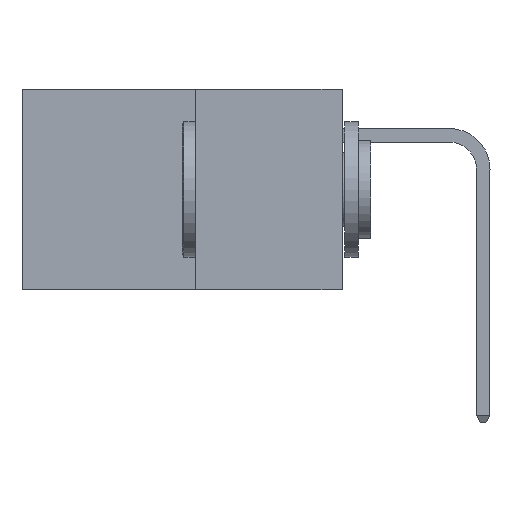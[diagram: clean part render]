
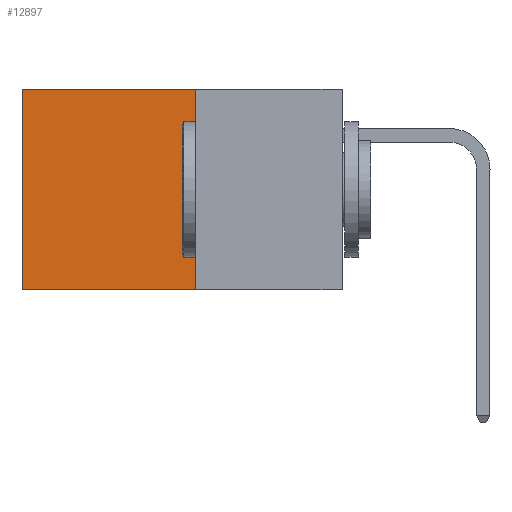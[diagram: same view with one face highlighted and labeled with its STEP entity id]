
A CAD part, left-side view. The second image highlights one B-rep face of the part: STEP entity #12897.
In plain terms, the highlighted planar face has unit normal (-1, 0, 0).
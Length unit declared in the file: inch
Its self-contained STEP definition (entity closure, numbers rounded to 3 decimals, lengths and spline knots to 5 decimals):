
#49 = EDGE_CURVE ( 'NONE', #3563, #13172, #6910, .T. ) ;
#600 = CARTESIAN_POINT ( 'NONE',  ( 0.277, 0.59, -0.37 ) ) ;
#800 = CARTESIAN_POINT ( 'NONE',  ( 0.277, 0.27, 0. ) ) ;
#1199 = ORIENTED_EDGE ( 'NONE', *, *, #7363, .F. ) ;
#1762 = LINE ( 'NONE', #2324, #5193 ) ;
#1766 = LINE ( 'NONE', #14304, #11670 ) ;
#1885 = AXIS2_PLACEMENT_3D ( 'NONE', #2661, #12996, #5249 ) ;
#2324 = CARTESIAN_POINT ( 'NONE',  ( 0.277, 0.27, -0.37 ) ) ;
#2379 = DIRECTION ( 'NONE',  ( 0., 1., 0. ) ) ;
#2661 = CARTESIAN_POINT ( 'NONE',  ( 0.277, 0.27, -0.37 ) ) ;
#2667 = DIRECTION ( 'NONE',  ( 0., 0., -1. ) ) ;
#2758 = ORIENTED_EDGE ( 'NONE', *, *, #15173, .F. ) ;
#3563 = VERTEX_POINT ( 'NONE', #11240 ) ;
#3900 = PLANE ( 'NONE',  #1885 ) ;
#5193 = VECTOR ( 'NONE', #2379, 39.37008 ) ;
#5249 = DIRECTION ( 'NONE',  ( 0., 0., -1. ) ) ;
#6542 = LINE ( 'NONE', #800, #13421 ) ;
#6910 = LINE ( 'NONE', #16074, #13760 ) ;
#7363 = EDGE_CURVE ( 'NONE', #12703, #13172, #1762, .T. ) ;
#8321 = CARTESIAN_POINT ( 'NONE',  ( 0.277, 0.27, 0. ) ) ;
#8359 = ORIENTED_EDGE ( 'NONE', *, *, #49, .T. ) ;
#8490 = ORIENTED_EDGE ( 'NONE', *, *, #9255, .T. ) ;
#8566 = DIRECTION ( 'NONE',  ( 0., 1., 0. ) ) ;
#9255 = EDGE_CURVE ( 'NONE', #13143, #3563, #6542, .T. ) ;
#11101 = DIRECTION ( 'NONE',  ( 0., 0., -1. ) ) ;
#11240 = CARTESIAN_POINT ( 'NONE',  ( 0.277, 0.59, 0. ) ) ;
#11670 = VECTOR ( 'NONE', #2667, 39.37008 ) ;
#12703 = VERTEX_POINT ( 'NONE', #16335 ) ;
#12897 = ADVANCED_FACE ( 'NONE', ( #13356 ), #3900, .F. ) ;
#12996 = DIRECTION ( 'NONE',  ( 1., 0., 0. ) ) ;
#13143 = VERTEX_POINT ( 'NONE', #8321 ) ;
#13172 = VERTEX_POINT ( 'NONE', #600 ) ;
#13356 = FACE_OUTER_BOUND ( 'NONE', #16064, .T. ) ;
#13421 = VECTOR ( 'NONE', #8566, 39.37008 ) ;
#13760 = VECTOR ( 'NONE', #11101, 39.37008 ) ;
#14304 = CARTESIAN_POINT ( 'NONE',  ( 0.277, 0.27, -0.37 ) ) ;
#15173 = EDGE_CURVE ( 'NONE', #13143, #12703, #1766, .T. ) ;
#16064 = EDGE_LOOP ( 'NONE', ( #8359, #1199, #2758, #8490 ) ) ;
#16074 = CARTESIAN_POINT ( 'NONE',  ( 0.277, 0.59, -0.37 ) ) ;
#16335 = CARTESIAN_POINT ( 'NONE',  ( 0.277, 0.27, -0.37 ) ) ;
